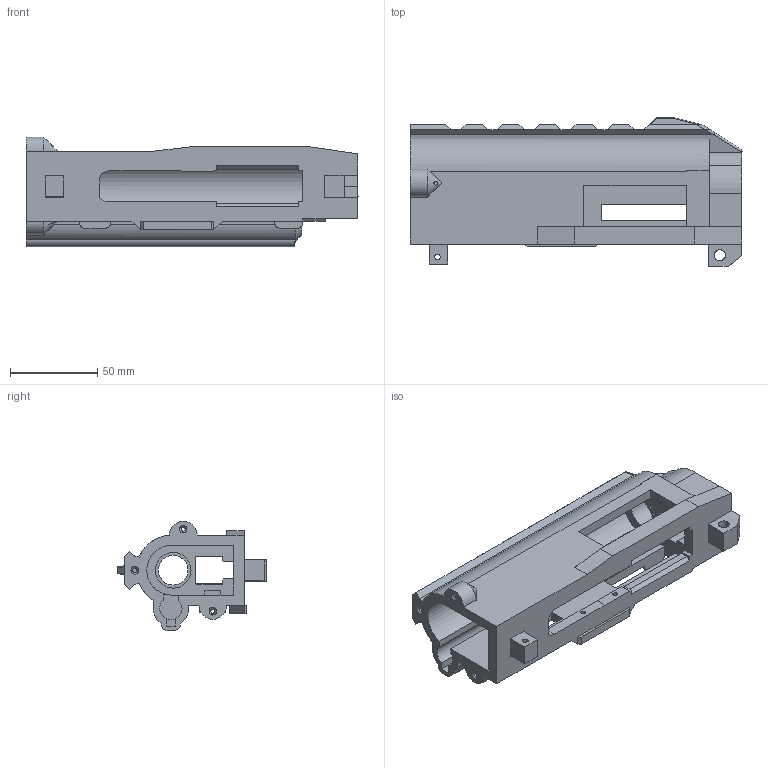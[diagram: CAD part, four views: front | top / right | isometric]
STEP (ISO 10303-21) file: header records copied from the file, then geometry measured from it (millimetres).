
FILE_DESCRIPTION (( 'STEP AP203' ), '1' );
FILE_NAME ('WTF-9H_upper_receiver.STEP', '2020-05-10T22:25:39', ( '' ), ( '' ), 'SwSTEP 2.0', 'SolidWorks 2016', '' );
FILE_SCHEMA (( 'CONFIG_CONTROL_DESIGN' ));
Length unit declared in the file: millimetre
Products named in the file (1): WTF-9H_upper_receiver
Bounding box: 190.38 x 85.37 x 62.82 mm (x, y, z)
Volume: 219609.6 mm3; surface area: 80296.5 mm2
Topology: 1 solids, 2 shells, 334 faces, 938 edges, 612 vertices
Faces by surface type: plane 267, cylinder 55, cone 10, sphere 2
Full cylindrical faces by diameter (mm): 2 x1, 2.2 x1, 2.4 x5, 2.5 x1, 2.6 x2, 3.175 x1, 6.375 x2, 17 x1, 20.49 x1
Entity records: 14001 total; most frequent: CARTESIAN_POINT 5533, ORIENTED_EDGE 1808, DIRECTION 1564, EDGE_CURVE 904, VECTOR 770, LINE 770, VERTEX_POINT 601, AXIS2_PLACEMENT_3D 397
